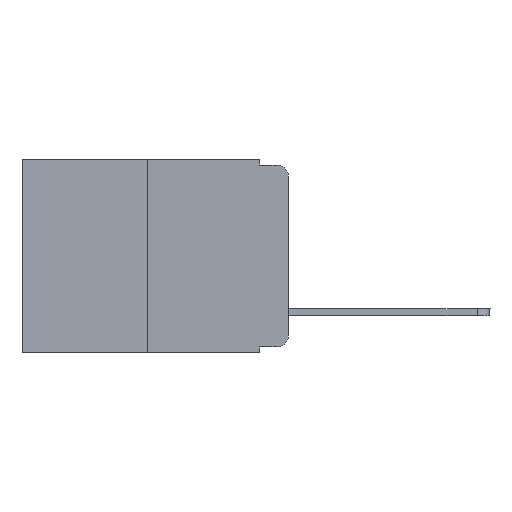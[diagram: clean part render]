
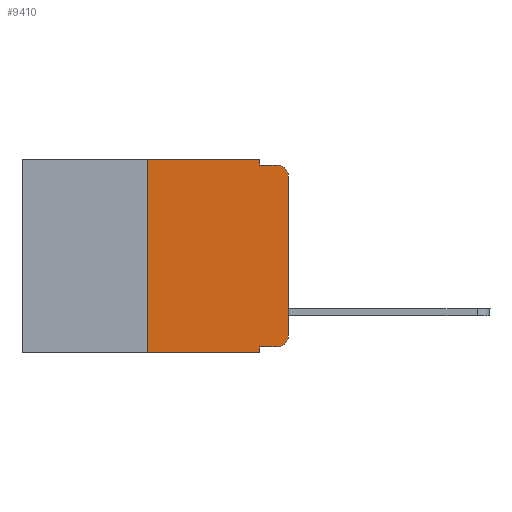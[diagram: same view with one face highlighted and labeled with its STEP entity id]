
A CAD part, left-side view. The second image highlights one B-rep face of the part: STEP entity #9410.
In plain terms, the highlighted planar face has unit normal (-1, 0, 0).
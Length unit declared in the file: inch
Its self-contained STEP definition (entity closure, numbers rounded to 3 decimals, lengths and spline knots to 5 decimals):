
#126 = EDGE_CURVE ( 'NONE', #9384, #4418, #13971, .T. ) ;
#468 = DIRECTION ( 'NONE',  ( -1., 0., 0. ) ) ;
#539 = DIRECTION ( 'NONE',  ( 0., -1., 0. ) ) ;
#645 = CARTESIAN_POINT ( 'NONE',  ( 0., 0.051, -0.343 ) ) ;
#748 = AXIS2_PLACEMENT_3D ( 'NONE', #9939, #468, #4592 ) ;
#892 = LINE ( 'NONE', #8518, #11212 ) ;
#1035 = CARTESIAN_POINT ( 'NONE',  ( 0., 0.051, -0.333 ) ) ;
#1173 = VERTEX_POINT ( 'NONE', #3411 ) ;
#1197 = CIRCLE ( 'NONE', #748, 0.02 ) ;
#1459 = LINE ( 'NONE', #11131, #12272 ) ;
#1709 = DIRECTION ( 'NONE',  ( 1., 0., 0. ) ) ;
#1856 = DIRECTION ( 'NONE',  ( 0., 0., -1. ) ) ;
#1872 = ORIENTED_EDGE ( 'NONE', *, *, #11871, .F. ) ;
#1902 = EDGE_CURVE ( 'NONE', #5714, #2215, #892, .T. ) ;
#2031 = LINE ( 'NONE', #3303, #10679 ) ;
#2107 = LINE ( 'NONE', #8673, #7226 ) ;
#2215 = VERTEX_POINT ( 'NONE', #4985 ) ;
#2241 = CARTESIAN_POINT ( 'NONE',  ( 0., 0., -0.313 ) ) ;
#2349 = ORIENTED_EDGE ( 'NONE', *, *, #10851, .T. ) ;
#2980 = VERTEX_POINT ( 'NONE', #11150 ) ;
#3007 = DIRECTION ( 'NONE',  ( 0., 0., -1. ) ) ;
#3044 = DIRECTION ( 'NONE',  ( 0., -1., 0. ) ) ;
#3303 = CARTESIAN_POINT ( 'NONE',  ( 0., 0.25, 0. ) ) ;
#3395 = EDGE_CURVE ( 'NONE', #8994, #4547, #1459, .T. ) ;
#3411 = CARTESIAN_POINT ( 'NONE',  ( 0., 0.25, 0. ) ) ;
#3434 = FACE_OUTER_BOUND ( 'NONE', #13231, .T. ) ;
#3568 = CARTESIAN_POINT ( 'NONE',  ( 0., 0.051, 0. ) ) ;
#3623 = VERTEX_POINT ( 'NONE', #7668 ) ;
#4072 = DIRECTION ( 'NONE',  ( -1., 0., 0. ) ) ;
#4301 = VECTOR ( 'NONE', #5361, 39.37008 ) ;
#4372 = DIRECTION ( 'NONE',  ( 0., -1., 0. ) ) ;
#4418 = VERTEX_POINT ( 'NONE', #5096 ) ;
#4547 = VERTEX_POINT ( 'NONE', #645 ) ;
#4592 = DIRECTION ( 'NONE',  ( 0., 0., -1. ) ) ;
#4985 = CARTESIAN_POINT ( 'NONE',  ( 0., 0., -0.03 ) ) ;
#5054 = CARTESIAN_POINT ( 'NONE',  ( 0., 0.051, 0. ) ) ;
#5096 = CARTESIAN_POINT ( 'NONE',  ( 0., 0.051, -0.01 ) ) ;
#5361 = DIRECTION ( 'NONE',  ( 0., -1., 0. ) ) ;
#5406 = ORIENTED_EDGE ( 'NONE', *, *, #13749, .T. ) ;
#5504 = LINE ( 'NONE', #1035, #4301 ) ;
#5659 = VECTOR ( 'NONE', #1856, 39.37008 ) ;
#5714 = VERTEX_POINT ( 'NONE', #2241 ) ;
#5856 = ORIENTED_EDGE ( 'NONE', *, *, #10546, .F. ) ;
#6352 = DIRECTION ( 'NONE',  ( 0., 0., 1. ) ) ;
#6908 = ORIENTED_EDGE ( 'NONE', *, *, #10013, .F. ) ;
#7123 = ORIENTED_EDGE ( 'NONE', *, *, #11889, .T. ) ;
#7133 = CARTESIAN_POINT ( 'NONE',  ( 0., 0.051, -0.01 ) ) ;
#7226 = VECTOR ( 'NONE', #4372, 39.37008 ) ;
#7668 = CARTESIAN_POINT ( 'NONE',  ( 0., 0.02, -0.333 ) ) ;
#7964 = AXIS2_PLACEMENT_3D ( 'NONE', #11047, #1709, #11307 ) ;
#8096 = VECTOR ( 'NONE', #11859, 39.37008 ) ;
#8518 = CARTESIAN_POINT ( 'NONE',  ( 0., 0., 0. ) ) ;
#8673 = CARTESIAN_POINT ( 'NONE',  ( 0., 0.473, 0. ) ) ;
#8714 = ORIENTED_EDGE ( 'NONE', *, *, #1902, .T. ) ;
#8994 = VERTEX_POINT ( 'NONE', #11065 ) ;
#9194 = VERTEX_POINT ( 'NONE', #12399 ) ;
#9384 = VERTEX_POINT ( 'NONE', #3568 ) ;
#9410 = ADVANCED_FACE ( 'NONE', ( #3434 ), #9921, .F. ) ;
#9421 = CARTESIAN_POINT ( 'NONE',  ( 0., 0.02, -0.313 ) ) ;
#9777 = DIRECTION ( 'NONE',  ( 0., 0., 1. ) ) ;
#9921 = PLANE ( 'NONE',  #7964 ) ;
#9939 = CARTESIAN_POINT ( 'NONE',  ( 0., 0.02, -0.03 ) ) ;
#10013 = EDGE_CURVE ( 'NONE', #4418, #2980, #12711, .T. ) ;
#10546 = EDGE_CURVE ( 'NONE', #8994, #1173, #2031, .T. ) ;
#10604 = ORIENTED_EDGE ( 'NONE', *, *, #3395, .T. ) ;
#10679 = VECTOR ( 'NONE', #6352, 39.37008 ) ;
#10851 = EDGE_CURVE ( 'NONE', #3623, #5714, #13283, .T. ) ;
#11047 = CARTESIAN_POINT ( 'NONE',  ( 0., 0.473, 0. ) ) ;
#11065 = CARTESIAN_POINT ( 'NONE',  ( 0., 0.25, -0.343 ) ) ;
#11131 = CARTESIAN_POINT ( 'NONE',  ( 0., 0.473, -0.343 ) ) ;
#11150 = CARTESIAN_POINT ( 'NONE',  ( 0., 0.02, -0.01 ) ) ;
#11212 = VECTOR ( 'NONE', #9777, 39.37008 ) ;
#11307 = DIRECTION ( 'NONE',  ( 0., 0., -1. ) ) ;
#11331 = ORIENTED_EDGE ( 'NONE', *, *, #12518, .F. ) ;
#11527 = LINE ( 'NONE', #5054, #5659 ) ;
#11859 = DIRECTION ( 'NONE',  ( 0., 0., -1. ) ) ;
#11871 = EDGE_CURVE ( 'NONE', #1173, #9384, #2107, .T. ) ;
#11889 = EDGE_CURVE ( 'NONE', #9194, #3623, #5504, .T. ) ;
#12272 = VECTOR ( 'NONE', #539, 39.37008 ) ;
#12399 = CARTESIAN_POINT ( 'NONE',  ( 0., 0.051, -0.333 ) ) ;
#12518 = EDGE_CURVE ( 'NONE', #9194, #4547, #11527, .T. ) ;
#12711 = LINE ( 'NONE', #7133, #13385 ) ;
#12716 = ORIENTED_EDGE ( 'NONE', *, *, #126, .F. ) ;
#12997 = CARTESIAN_POINT ( 'NONE',  ( 0., 0.051, 0. ) ) ;
#13061 = AXIS2_PLACEMENT_3D ( 'NONE', #9421, #4072, #3007 ) ;
#13231 = EDGE_LOOP ( 'NONE', ( #8714, #5406, #6908, #12716, #1872, #5856, #10604, #11331, #7123, #2349 ) ) ;
#13283 = CIRCLE ( 'NONE', #13061, 0.02 ) ;
#13385 = VECTOR ( 'NONE', #3044, 39.37008 ) ;
#13749 = EDGE_CURVE ( 'NONE', #2215, #2980, #1197, .T. ) ;
#13971 = LINE ( 'NONE', #12997, #8096 ) ;
